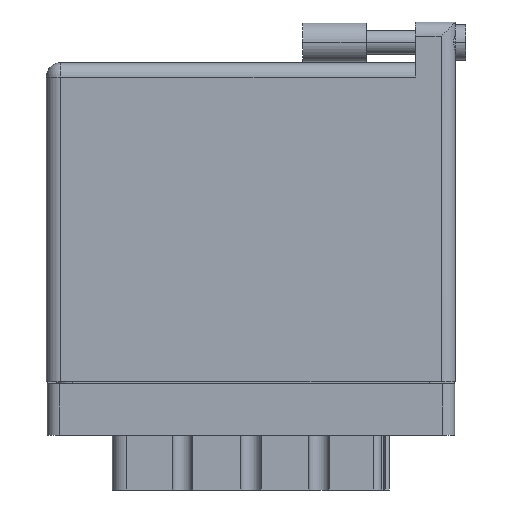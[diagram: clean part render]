
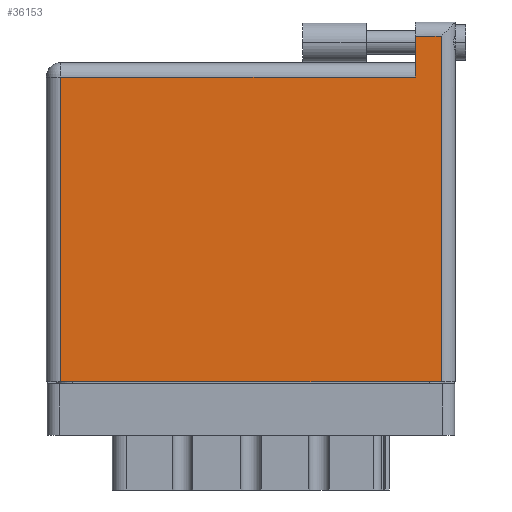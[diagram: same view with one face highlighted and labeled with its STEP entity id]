
A CAD part, front view. The second image highlights one B-rep face of the part: STEP entity #36153.
In plain terms, the highlighted face is planar.
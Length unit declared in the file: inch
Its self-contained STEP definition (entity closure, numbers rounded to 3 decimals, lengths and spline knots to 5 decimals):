
#1268 = VERTEX_POINT ( 'NONE', #4337 ) ;
#2044 = DIRECTION ( 'NONE',  ( 0., -1., 0. ) ) ;
#2059 = LINE ( 'NONE', #32101, #32795 ) ;
#2130 = ORIENTED_EDGE ( 'NONE', *, *, #16781, .T. ) ;
#4337 = CARTESIAN_POINT ( 'NONE',  ( 1.811, 1.496, 0. ) ) ;
#7400 = CARTESIAN_POINT ( 'NONE',  ( 1.811, 1.696, 0. ) ) ;
#7656 = CARTESIAN_POINT ( 'NONE',  ( 1.938, 1.766, 0. ) ) ;
#7871 = CARTESIAN_POINT ( 'NONE',  ( 0., 0., 0. ) ) ;
#8612 = PLANE ( 'NONE',  #17717 ) ;
#9475 = DIRECTION ( 'NONE',  ( -1., 0., 0. ) ) ;
#11128 = DIRECTION ( 'NONE',  ( -1., 0., 0. ) ) ;
#12098 = VERTEX_POINT ( 'NONE', #14556 ) ;
#13152 = LINE ( 'NONE', #32816, #28271 ) ;
#13294 = ORIENTED_EDGE ( 'NONE', *, *, #14617, .T. ) ;
#13594 = ORIENTED_EDGE ( 'NONE', *, *, #18878, .T. ) ;
#14230 = DIRECTION ( 'NONE',  ( 0., 0., -1. ) ) ;
#14556 = CARTESIAN_POINT ( 'NONE',  ( 0.07, 1.496, 0. ) ) ;
#14617 = EDGE_CURVE ( 'NONE', #32589, #19364, #2059, .T. ) ;
#15808 = LINE ( 'NONE', #19138, #26454 ) ;
#16781 = EDGE_CURVE ( 'NONE', #1268, #12098, #13152, .T. ) ;
#17717 = AXIS2_PLACEMENT_3D ( 'NONE', #33891, #14230, #11128 ) ;
#18878 = EDGE_CURVE ( 'NONE', #19364, #1268, #31228, .T. ) ;
#19138 = CARTESIAN_POINT ( 'NONE',  ( 0.07, 0., 0. ) ) ;
#19364 = VERTEX_POINT ( 'NONE', #7400 ) ;
#19800 = LINE ( 'NONE', #7656, #26452 ) ;
#21756 = DIRECTION ( 'NONE',  ( -1., 0., 0. ) ) ;
#21903 = ORIENTED_EDGE ( 'NONE', *, *, #24907, .T. ) ;
#22356 = CARTESIAN_POINT ( 'NONE',  ( 1.938, 0., 0. ) ) ;
#22429 = EDGE_CURVE ( 'NONE', #12098, #34729, #15808, .T. ) ;
#22993 = EDGE_LOOP ( 'NONE', ( #30001, #21903, #13294, #13594, #2130, #31507 ) ) ;
#23498 = EDGE_CURVE ( 'NONE', #34729, #32168, #35356, .T. ) ;
#23665 = VECTOR ( 'NONE', #27855, 39.37008 ) ;
#24907 = EDGE_CURVE ( 'NONE', #32168, #32589, #19800, .T. ) ;
#26452 = VECTOR ( 'NONE', #33167, 39.37008 ) ;
#26454 = VECTOR ( 'NONE', #2044, 39.37008 ) ;
#27855 = DIRECTION ( 'NONE',  ( 0., -1., 0. ) ) ;
#28271 = VECTOR ( 'NONE', #21756, 39.37008 ) ;
#29168 = FACE_OUTER_BOUND ( 'NONE', #22993, .T. ) ;
#30001 = ORIENTED_EDGE ( 'NONE', *, *, #23498, .T. ) ;
#30566 = CARTESIAN_POINT ( 'NONE',  ( 1.811, 1.766, 0. ) ) ;
#30620 = CARTESIAN_POINT ( 'NONE',  ( 0.07, 0., 0. ) ) ;
#31228 = LINE ( 'NONE', #30566, #23665 ) ;
#31507 = ORIENTED_EDGE ( 'NONE', *, *, #22429, .T. ) ;
#31787 = VECTOR ( 'NONE', #35986, 39.37008 ) ;
#32101 = CARTESIAN_POINT ( 'NONE',  ( 0., 1.696, 0. ) ) ;
#32127 = CARTESIAN_POINT ( 'NONE',  ( 1.938, 1.696, 0. ) ) ;
#32168 = VERTEX_POINT ( 'NONE', #22356 ) ;
#32589 = VERTEX_POINT ( 'NONE', #32127 ) ;
#32795 = VECTOR ( 'NONE', #9475, 39.37008 ) ;
#32816 = CARTESIAN_POINT ( 'NONE',  ( 0., 1.496, 0. ) ) ;
#33167 = DIRECTION ( 'NONE',  ( 0., 1., 0. ) ) ;
#33891 = CARTESIAN_POINT ( 'NONE',  ( 0., 1.566, 0. ) ) ;
#34729 = VERTEX_POINT ( 'NONE', #30620 ) ;
#35356 = LINE ( 'NONE', #7871, #31787 ) ;
#35986 = DIRECTION ( 'NONE',  ( 1., 0., 0. ) ) ;
#36153 = ADVANCED_FACE ( 'NONE', ( #29168 ), #8612, .F. ) ;
